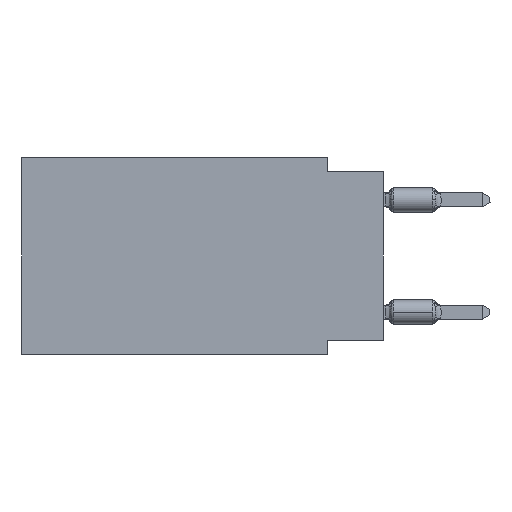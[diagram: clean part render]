
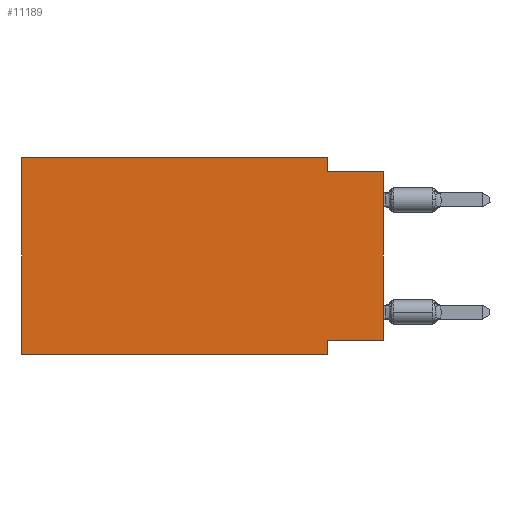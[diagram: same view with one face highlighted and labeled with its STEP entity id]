
A CAD part, left-side view. The second image highlights one B-rep face of the part: STEP entity #11189.
In plain terms, the highlighted planar face has unit normal (-1, 0, 0).
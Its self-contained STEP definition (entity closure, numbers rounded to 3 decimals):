
#610 = VECTOR ( 'NONE', #23683, 1000. ) ;
#949 = CARTESIAN_POINT ( 'NONE',  ( 0., 2.54, 0. ) ) ;
#2773 = LINE ( 'NONE', #24448, #11104 ) ;
#2952 = DIRECTION ( 'NONE',  ( 0., 0., 1. ) ) ;
#3133 = CARTESIAN_POINT ( 'NONE',  ( 0., 0., -0.635 ) ) ;
#3157 = LINE ( 'NONE', #21582, #24677 ) ;
#3580 = FACE_OUTER_BOUND ( 'NONE', #11648, .T. ) ;
#5172 = DIRECTION ( 'NONE',  ( 0., 0., -1. ) ) ;
#5917 = EDGE_CURVE ( 'NONE', #17938, #17992, #22357, .T. ) ;
#6811 = DIRECTION ( 'NONE',  ( 0., 0., 1. ) ) ;
#6911 = CARTESIAN_POINT ( 'NONE',  ( 0., 16.383, -8.89 ) ) ;
#7264 = VERTEX_POINT ( 'NONE', #19792 ) ;
#8233 = VECTOR ( 'NONE', #6811, 1000. ) ;
#9397 = VERTEX_POINT ( 'NONE', #32593 ) ;
#10277 = VECTOR ( 'NONE', #5172, 1000. ) ;
#10566 = LINE ( 'NONE', #949, #28077 ) ;
#11104 = VECTOR ( 'NONE', #36765, 1000. ) ;
#11189 = ADVANCED_FACE ( 'NONE', ( #3580 ), #24877, .F. ) ;
#11648 = EDGE_LOOP ( 'NONE', ( #20030, #17808, #35440, #33770, #23293, #30712, #36694, #15367 ) ) ;
#12594 = DIRECTION ( 'NONE',  ( 0., 0., -1. ) ) ;
#13728 = VECTOR ( 'NONE', #17139, 1000. ) ;
#14272 = CARTESIAN_POINT ( 'NONE',  ( 0., 16.383, 0. ) ) ;
#15367 = ORIENTED_EDGE ( 'NONE', *, *, #38368, .F. ) ;
#17139 = DIRECTION ( 'NONE',  ( 0., 1., 0. ) ) ;
#17808 = ORIENTED_EDGE ( 'NONE', *, *, #5917, .F. ) ;
#17938 = VERTEX_POINT ( 'NONE', #18671 ) ;
#17992 = VERTEX_POINT ( 'NONE', #28889 ) ;
#18219 = VERTEX_POINT ( 'NONE', #23767 ) ;
#18671 = CARTESIAN_POINT ( 'NONE',  ( 0., 2.54, -0.635 ) ) ;
#18799 = VERTEX_POINT ( 'NONE', #32084 ) ;
#19792 = CARTESIAN_POINT ( 'NONE',  ( 0., 2.54, -8.89 ) ) ;
#20030 = ORIENTED_EDGE ( 'NONE', *, *, #32376, .T. ) ;
#21268 = EDGE_CURVE ( 'NONE', #18799, #17938, #10566, .T. ) ;
#21509 = EDGE_CURVE ( 'NONE', #28139, #7264, #2773, .T. ) ;
#21582 = CARTESIAN_POINT ( 'NONE',  ( 0., 16.383, 0. ) ) ;
#22162 = LINE ( 'NONE', #34877, #8233 ) ;
#22357 = LINE ( 'NONE', #3133, #37110 ) ;
#23293 = ORIENTED_EDGE ( 'NONE', *, *, #30251, .F. ) ;
#23458 = CARTESIAN_POINT ( 'NONE',  ( 0., 0., -8.255 ) ) ;
#23683 = DIRECTION ( 'NONE',  ( 0., -1., 0. ) ) ;
#23767 = CARTESIAN_POINT ( 'NONE',  ( 0., 0., -8.255 ) ) ;
#24079 = LINE ( 'NONE', #14272, #610 ) ;
#24448 = CARTESIAN_POINT ( 'NONE',  ( 0., 16.383, -8.89 ) ) ;
#24677 = VECTOR ( 'NONE', #2952, 1000. ) ;
#24877 = PLANE ( 'NONE',  #39080 ) ;
#25037 = VERTEX_POINT ( 'NONE', #31804 ) ;
#27185 = EDGE_CURVE ( 'NONE', #9397, #18799, #24079, .T. ) ;
#28077 = VECTOR ( 'NONE', #34749, 1000. ) ;
#28139 = VERTEX_POINT ( 'NONE', #6911 ) ;
#28546 = DIRECTION ( 'NONE',  ( 1., 0., 0. ) ) ;
#28889 = CARTESIAN_POINT ( 'NONE',  ( 0., 0., -0.635 ) ) ;
#30251 = EDGE_CURVE ( 'NONE', #28139, #9397, #3157, .T. ) ;
#30712 = ORIENTED_EDGE ( 'NONE', *, *, #21509, .T. ) ;
#31804 = CARTESIAN_POINT ( 'NONE',  ( 0., 2.54, -8.255 ) ) ;
#32084 = CARTESIAN_POINT ( 'NONE',  ( 0., 2.54, 0. ) ) ;
#32376 = EDGE_CURVE ( 'NONE', #18219, #17992, #22162, .T. ) ;
#32480 = LINE ( 'NONE', #23458, #13728 ) ;
#32593 = CARTESIAN_POINT ( 'NONE',  ( 0., 16.383, 0. ) ) ;
#33226 = CARTESIAN_POINT ( 'NONE',  ( 0., 2.54, -8.89 ) ) ;
#33770 = ORIENTED_EDGE ( 'NONE', *, *, #27185, .F. ) ;
#33891 = EDGE_CURVE ( 'NONE', #25037, #7264, #36284, .T. ) ;
#34302 = CARTESIAN_POINT ( 'NONE',  ( 0., 16.383, 0. ) ) ;
#34749 = DIRECTION ( 'NONE',  ( 0., 0., -1. ) ) ;
#34877 = CARTESIAN_POINT ( 'NONE',  ( 0., 0., 0. ) ) ;
#35064 = DIRECTION ( 'NONE',  ( 0., -1., 0. ) ) ;
#35440 = ORIENTED_EDGE ( 'NONE', *, *, #21268, .F. ) ;
#36284 = LINE ( 'NONE', #33226, #10277 ) ;
#36694 = ORIENTED_EDGE ( 'NONE', *, *, #33891, .F. ) ;
#36765 = DIRECTION ( 'NONE',  ( 0., -1., 0. ) ) ;
#37110 = VECTOR ( 'NONE', #35064, 1000. ) ;
#38368 = EDGE_CURVE ( 'NONE', #18219, #25037, #32480, .T. ) ;
#39080 = AXIS2_PLACEMENT_3D ( 'NONE', #34302, #28546, #12594 ) ;
